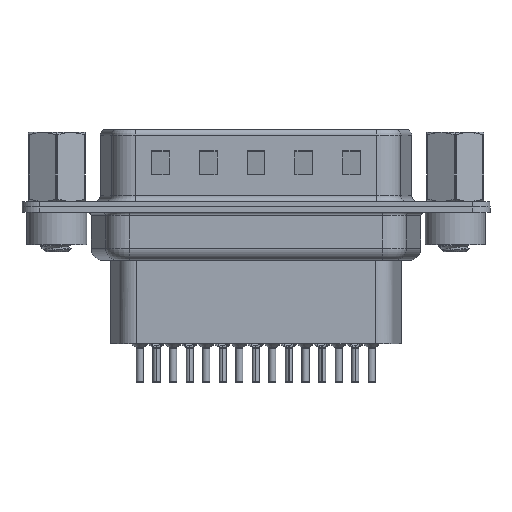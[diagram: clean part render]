
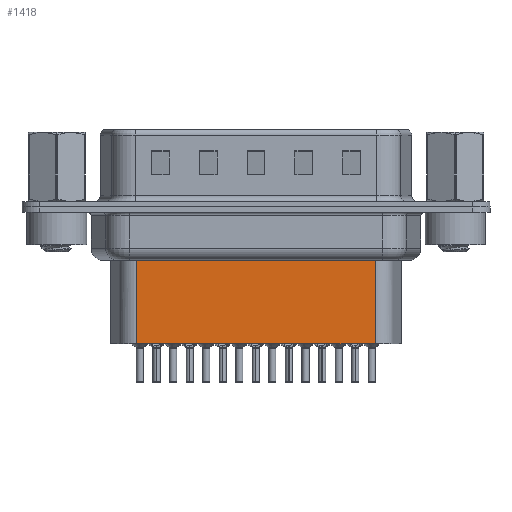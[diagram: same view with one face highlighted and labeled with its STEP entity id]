
A CAD part, front view. The second image highlights one B-rep face of the part: STEP entity #1418.
In plain terms, the highlighted planar face has unit normal (0, -1, 0).
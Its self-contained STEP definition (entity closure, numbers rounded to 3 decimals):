
#256 = VERTEX_POINT ( 'NONE', #5434 ) ;
#493 = CARTESIAN_POINT ( 'NONE',  ( 6.681, -3.5, -3.1 ) ) ;
#1418 = ADVANCED_FACE ( 'NONE', ( #2702 ), #24754, .T. ) ;
#1846 = DIRECTION ( 'NONE',  ( 0., 0., -1. ) ) ;
#2044 = CARTESIAN_POINT ( 'NONE',  ( 6.434, -3.5, -4.097 ) ) ;
#2702 = FACE_OUTER_BOUND ( 'NONE', #9343, .T. ) ;
#2927 = AXIS2_PLACEMENT_3D ( 'NONE', #493, #25484, #25419 ) ;
#3495 = EDGE_CURVE ( 'NONE', #256, #24773, #21085, .T. ) ;
#4501 = ORIENTED_EDGE ( 'NONE', *, *, #16212, .F. ) ;
#4609 = ORIENTED_EDGE ( 'NONE', *, *, #11673, .T. ) ;
#5434 = CARTESIAN_POINT ( 'NONE',  ( 26.619, -3.5, -4.097 ) ) ;
#5729 = VECTOR ( 'NONE', #24241, 1000. ) ;
#5764 = LINE ( 'NONE', #23724, #15831 ) ;
#6111 = VERTEX_POINT ( 'NONE', #16697 ) ;
#8322 = VECTOR ( 'NONE', #1846, 1000. ) ;
#9065 = ORIENTED_EDGE ( 'NONE', *, *, #10792, .F. ) ;
#9343 = EDGE_LOOP ( 'NONE', ( #9065, #21621, #4609, #4501 ) ) ;
#10102 = DIRECTION ( 'NONE',  ( -1., 0., 0. ) ) ;
#10792 = EDGE_CURVE ( 'NONE', #256, #11792, #24323, .T. ) ;
#11673 = EDGE_CURVE ( 'NONE', #24773, #6111, #5764, .T. ) ;
#11792 = VERTEX_POINT ( 'NONE', #20211 ) ;
#11872 = CARTESIAN_POINT ( 'NONE',  ( 26.619, -3.5, -3.1 ) ) ;
#15831 = VECTOR ( 'NONE', #25757, 1000. ) ;
#15897 = VECTOR ( 'NONE', #10102, 1000. ) ;
#16202 = CARTESIAN_POINT ( 'NONE',  ( 6.681, -3.5, -11.45 ) ) ;
#16212 = EDGE_CURVE ( 'NONE', #11792, #6111, #20590, .T. ) ;
#16697 = CARTESIAN_POINT ( 'NONE',  ( 6.681, -3.5, -11.45 ) ) ;
#20211 = CARTESIAN_POINT ( 'NONE',  ( 26.619, -3.5, -11.45 ) ) ;
#20590 = LINE ( 'NONE', #16202, #15897 ) ;
#21085 = LINE ( 'NONE', #2044, #5729 ) ;
#21621 = ORIENTED_EDGE ( 'NONE', *, *, #3495, .T. ) ;
#22782 = CARTESIAN_POINT ( 'NONE',  ( 6.681, -3.5, -4.097 ) ) ;
#23724 = CARTESIAN_POINT ( 'NONE',  ( 6.681, -3.5, -3.1 ) ) ;
#24241 = DIRECTION ( 'NONE',  ( -1., 0., 0. ) ) ;
#24323 = LINE ( 'NONE', #11872, #8322 ) ;
#24754 = PLANE ( 'NONE',  #2927 ) ;
#24773 = VERTEX_POINT ( 'NONE', #22782 ) ;
#25419 = DIRECTION ( 'NONE',  ( 1., 0., 0. ) ) ;
#25484 = DIRECTION ( 'NONE',  ( 0., -1., 0. ) ) ;
#25757 = DIRECTION ( 'NONE',  ( 0., 0., -1. ) ) ;
